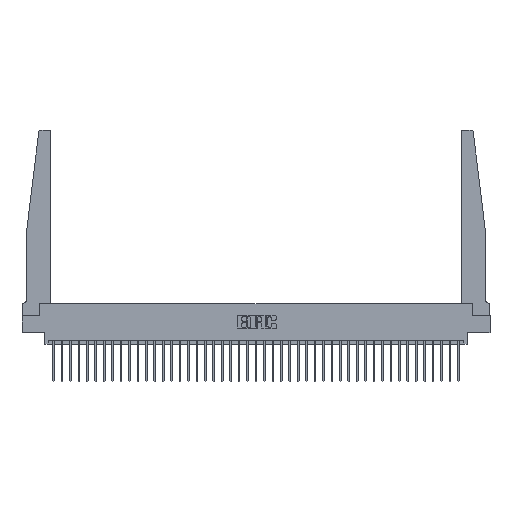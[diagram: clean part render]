
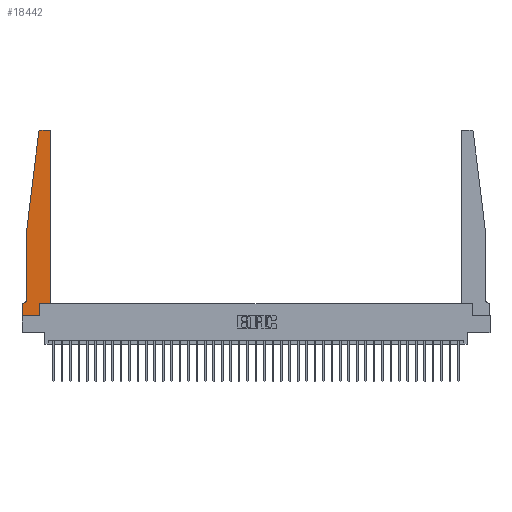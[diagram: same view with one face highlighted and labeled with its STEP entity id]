
A CAD part, top view. The second image highlights one B-rep face of the part: STEP entity #18442.
In plain terms, the highlighted planar face has unit normal (0, 0, 1).
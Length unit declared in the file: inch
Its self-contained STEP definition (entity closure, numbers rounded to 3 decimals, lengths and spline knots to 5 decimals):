
#131 = VERTEX_POINT ( 'NONE', #7978 ) ;
#414 = PLANE ( 'NONE',  #7101 ) ;
#473 = EDGE_CURVE ( 'NONE', #11662, #12091, #2344, .T. ) ;
#680 = ORIENTED_EDGE ( 'NONE', *, *, #1773, .T. ) ;
#990 = LINE ( 'NONE', #15535, #9694 ) ;
#1470 = CARTESIAN_POINT ( 'NONE',  ( 0., 0., 0.37 ) ) ;
#1773 = EDGE_CURVE ( 'NONE', #27223, #34399, #24659, .T. ) ;
#1814 = DIRECTION ( 'NONE',  ( -0.122, -0.992, 0. ) ) ;
#2344 = LINE ( 'NONE', #25014, #28651 ) ;
#2353 = VECTOR ( 'NONE', #12976, 39.37008 ) ;
#2619 = DIRECTION ( 'NONE',  ( 0., 0., 1. ) ) ;
#2737 = ORIENTED_EDGE ( 'NONE', *, *, #17006, .T. ) ;
#3127 = CARTESIAN_POINT ( 'NONE',  ( 0.395, 2.72, 0.37 ) ) ;
#3167 = CARTESIAN_POINT ( 'NONE',  ( 0., 0.1875, 0.37 ) ) ;
#3307 = CARTESIAN_POINT ( 'NONE',  ( 0.395, 2.75, 0.37 ) ) ;
#3405 = CARTESIAN_POINT ( 'NONE',  ( 0.065, 0.2375, 0.37 ) ) ;
#3412 = DIRECTION ( 'NONE',  ( 0., 0., 1. ) ) ;
#3921 = CIRCLE ( 'NONE', #28080, 0.03 ) ;
#5741 = DIRECTION ( 'NONE',  ( 1., 0., 0. ) ) ;
#6051 = VECTOR ( 'NONE', #1814, 39.37008 ) ;
#6149 = CARTESIAN_POINT ( 'NONE',  ( 0., 0., 0.37 ) ) ;
#7101 = AXIS2_PLACEMENT_3D ( 'NONE', #3167, #2619, #5741 ) ;
#7890 = ORIENTED_EDGE ( 'NONE', *, *, #27152, .T. ) ;
#7978 = CARTESIAN_POINT ( 'NONE',  ( 0.015, 0.1875, 0.37 ) ) ;
#8885 = EDGE_CURVE ( 'NONE', #21669, #32399, #9927, .T. ) ;
#8919 = AXIS2_PLACEMENT_3D ( 'NONE', #14640, #3412, #34180 ) ;
#9135 = VERTEX_POINT ( 'NONE', #33625 ) ;
#9223 = CARTESIAN_POINT ( 'NONE',  ( 0., 0.1875, 0.37 ) ) ;
#9503 = CIRCLE ( 'NONE', #8919, 0.03 ) ;
#9559 = VERTEX_POINT ( 'NONE', #21806 ) ;
#9580 = ORIENTED_EDGE ( 'NONE', *, *, #23852, .T. ) ;
#9694 = VECTOR ( 'NONE', #18492, 39.37008 ) ;
#9737 = CARTESIAN_POINT ( 'NONE',  ( 0.425, 0.18, 0.37 ) ) ;
#9847 = VERTEX_POINT ( 'NONE', #32289 ) ;
#9927 = LINE ( 'NONE', #1470, #14806 ) ;
#10203 = CARTESIAN_POINT ( 'NONE',  ( 0.25, 2.75, 0.37 ) ) ;
#11662 = VERTEX_POINT ( 'NONE', #9737 ) ;
#11723 = DIRECTION ( 'NONE',  ( 1., 0., 0. ) ) ;
#12091 = VERTEX_POINT ( 'NONE', #20577 ) ;
#12644 = CARTESIAN_POINT ( 'NONE',  ( 0.015, 0.2375, 0.37 ) ) ;
#12976 = DIRECTION ( 'NONE',  ( -1., 0., 0. ) ) ;
#14491 = LINE ( 'NONE', #26128, #26599 ) ;
#14640 = CARTESIAN_POINT ( 'NONE',  ( 0.27653, 2.72, 0.37 ) ) ;
#14806 = VECTOR ( 'NONE', #23978, 39.37008 ) ;
#15535 = CARTESIAN_POINT ( 'NONE',  ( 0.065, 0.1875, 0.37 ) ) ;
#15572 = LINE ( 'NONE', #10203, #2353 ) ;
#16045 = VECTOR ( 'NONE', #24198, 39.37008 ) ;
#17006 = EDGE_CURVE ( 'NONE', #34616, #9559, #15572, .T. ) ;
#18442 = ADVANCED_FACE ( 'NONE', ( #28419 ), #414, .T. ) ;
#18492 = DIRECTION ( 'NONE',  ( -1., 0., 0. ) ) ;
#19111 = DIRECTION ( 'NONE',  ( 0., 1., 0. ) ) ;
#19460 = ORIENTED_EDGE ( 'NONE', *, *, #35353, .T. ) ;
#19517 = DIRECTION ( 'NONE',  ( 1., 0., 0. ) ) ;
#19800 = CARTESIAN_POINT ( 'NONE',  ( 0.065, 1.25, 0.37 ) ) ;
#20577 = CARTESIAN_POINT ( 'NONE',  ( 0.425, 2.72, 0.37 ) ) ;
#20669 = DIRECTION ( 'NONE',  ( 0., -1., 0. ) ) ;
#21191 = ORIENTED_EDGE ( 'NONE', *, *, #473, .T. ) ;
#21411 = CARTESIAN_POINT ( 'NONE',  ( 0.065, 1.25, 0.37 ) ) ;
#21669 = VERTEX_POINT ( 'NONE', #9223 ) ;
#21806 = CARTESIAN_POINT ( 'NONE',  ( 0.27653, 2.75, 0.37 ) ) ;
#23852 = EDGE_CURVE ( 'NONE', #32399, #9847, #14491, .T. ) ;
#23978 = DIRECTION ( 'NONE',  ( 0., -1., 0. ) ) ;
#24026 = LINE ( 'NONE', #35256, #16045 ) ;
#24159 = EDGE_CURVE ( 'NONE', #9559, #27223, #9503, .T. ) ;
#24183 = LINE ( 'NONE', #21411, #31635 ) ;
#24198 = DIRECTION ( 'NONE',  ( 0., 1., 0. ) ) ;
#24274 = ORIENTED_EDGE ( 'NONE', *, *, #32900, .T. ) ;
#24659 = LINE ( 'NONE', #30380, #6051 ) ;
#24909 = DIRECTION ( 'NONE',  ( 1., 0., 0. ) ) ;
#25014 = CARTESIAN_POINT ( 'NONE',  ( 0.425, 0.18, 0.37 ) ) ;
#25616 = DIRECTION ( 'NONE',  ( 0., 0., 1. ) ) ;
#25838 = ORIENTED_EDGE ( 'NONE', *, *, #24159, .T. ) ;
#26128 = CARTESIAN_POINT ( 'NONE',  ( 0., 0., 0.37 ) ) ;
#26592 = ORIENTED_EDGE ( 'NONE', *, *, #29910, .T. ) ;
#26599 = VECTOR ( 'NONE', #11723, 39.37008 ) ;
#26998 = EDGE_CURVE ( 'NONE', #9847, #9135, #24026, .T. ) ;
#27152 = EDGE_CURVE ( 'NONE', #9135, #11662, #35973, .T. ) ;
#27223 = VERTEX_POINT ( 'NONE', #28579 ) ;
#28080 = AXIS2_PLACEMENT_3D ( 'NONE', #3127, #25616, #19517 ) ;
#28419 = FACE_OUTER_BOUND ( 'NONE', #32270, .T. ) ;
#28579 = CARTESIAN_POINT ( 'NONE',  ( 0.24675, 2.72367, 0.37 ) ) ;
#28584 = ORIENTED_EDGE ( 'NONE', *, *, #31998, .T. ) ;
#28651 = VECTOR ( 'NONE', #19111, 39.37008 ) ;
#29138 = ORIENTED_EDGE ( 'NONE', *, *, #8885, .T. ) ;
#29799 = DIRECTION ( 'NONE',  ( 0., 0., -1. ) ) ;
#29910 = EDGE_CURVE ( 'NONE', #131, #21669, #990, .T. ) ;
#30033 = ORIENTED_EDGE ( 'NONE', *, *, #26998, .T. ) ;
#30380 = CARTESIAN_POINT ( 'NONE',  ( 0.065, 1.25, 0.37 ) ) ;
#30503 = CIRCLE ( 'NONE', #34019, 0.05 ) ;
#31635 = VECTOR ( 'NONE', #20669, 39.37008 ) ;
#31998 = EDGE_CURVE ( 'NONE', #12091, #34616, #3921, .T. ) ;
#32270 = EDGE_LOOP ( 'NONE', ( #2737, #25838, #680, #24274, #19460, #26592, #29138, #9580, #30033, #7890, #21191, #28584 ) ) ;
#32289 = CARTESIAN_POINT ( 'NONE',  ( 0.2605, 0., 0.37 ) ) ;
#32399 = VERTEX_POINT ( 'NONE', #6149 ) ;
#32400 = VERTEX_POINT ( 'NONE', #3405 ) ;
#32900 = EDGE_CURVE ( 'NONE', #34399, #32400, #24183, .T. ) ;
#33625 = CARTESIAN_POINT ( 'NONE',  ( 0.2605, 0.18, 0.37 ) ) ;
#34019 = AXIS2_PLACEMENT_3D ( 'NONE', #12644, #29799, #35154 ) ;
#34180 = DIRECTION ( 'NONE',  ( 1., 0., 0. ) ) ;
#34399 = VERTEX_POINT ( 'NONE', #19800 ) ;
#34616 = VERTEX_POINT ( 'NONE', #3307 ) ;
#34902 = VECTOR ( 'NONE', #24909, 39.37008 ) ;
#35154 = DIRECTION ( 'NONE',  ( -1., 0., 0. ) ) ;
#35256 = CARTESIAN_POINT ( 'NONE',  ( 0.2605, 0.18, 0.37 ) ) ;
#35353 = EDGE_CURVE ( 'NONE', #32400, #131, #30503, .T. ) ;
#35619 = CARTESIAN_POINT ( 'NONE',  ( 0.425, 0.18, 0.37 ) ) ;
#35973 = LINE ( 'NONE', #35619, #34902 ) ;
